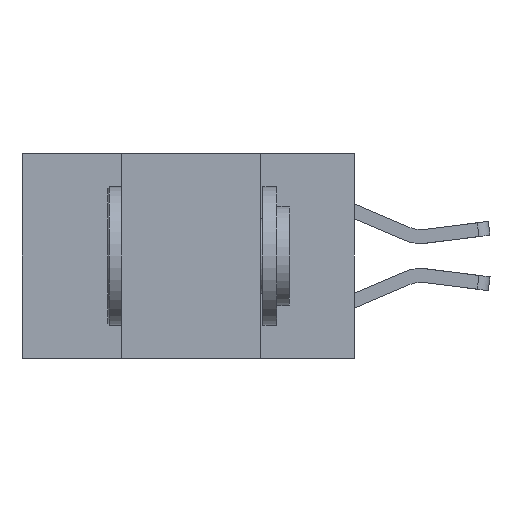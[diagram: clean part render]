
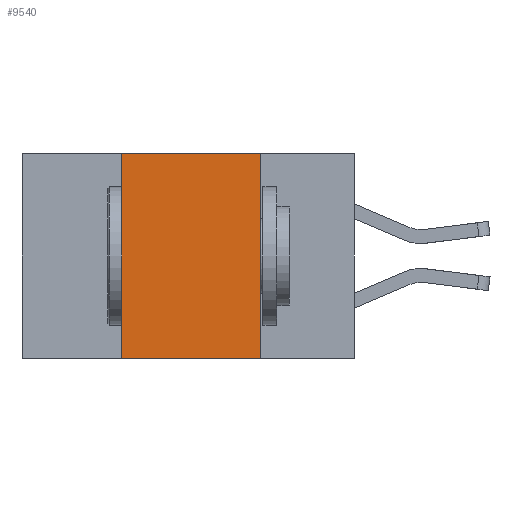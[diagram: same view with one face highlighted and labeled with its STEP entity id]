
A CAD part, left-side view. The second image highlights one B-rep face of the part: STEP entity #9540.
In plain terms, the highlighted planar face has unit normal (-1, 0, 0).
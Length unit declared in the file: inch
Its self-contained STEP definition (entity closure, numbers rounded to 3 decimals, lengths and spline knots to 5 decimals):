
#152 = EDGE_CURVE ( 'NONE', #859, #7637, #5741, .T. ) ;
#662 = EDGE_LOOP ( 'NONE', ( #2563, #6966, #4535, #7061 ) ) ;
#859 = VERTEX_POINT ( 'NONE', #6624 ) ;
#1360 = EDGE_CURVE ( 'NONE', #7637, #4985, #1801, .T. ) ;
#1801 = LINE ( 'NONE', #8387, #7916 ) ;
#1902 = LINE ( 'NONE', #7557, #3897 ) ;
#2563 = ORIENTED_EDGE ( 'NONE', *, *, #4761, .F. ) ;
#2686 = CARTESIAN_POINT ( 'NONE',  ( 0., 0.6, 0. ) ) ;
#2719 = DIRECTION ( 'NONE',  ( 0., 0., -1. ) ) ;
#2731 = AXIS2_PLACEMENT_3D ( 'NONE', #2686, #7675, #2719 ) ;
#3028 = EDGE_CURVE ( 'NONE', #859, #6926, #1902, .T. ) ;
#3897 = VECTOR ( 'NONE', #7527, 39.37008 ) ;
#4080 = VECTOR ( 'NONE', #9337, 39.37008 ) ;
#4535 = ORIENTED_EDGE ( 'NONE', *, *, #152, .F. ) ;
#4761 = EDGE_CURVE ( 'NONE', #4985, #6926, #6246, .T. ) ;
#4819 = DIRECTION ( 'NONE',  ( 0., 0., 1. ) ) ;
#4985 = VERTEX_POINT ( 'NONE', #6222 ) ;
#5354 = DIRECTION ( 'NONE',  ( 0., -1., 0. ) ) ;
#5741 = LINE ( 'NONE', #10121, #7667 ) ;
#6222 = CARTESIAN_POINT ( 'NONE',  ( 0., 0.17, 0. ) ) ;
#6246 = LINE ( 'NONE', #9583, #4080 ) ;
#6279 = CARTESIAN_POINT ( 'NONE',  ( 0., 0.42, 0. ) ) ;
#6624 = CARTESIAN_POINT ( 'NONE',  ( 0., 0.42, -0.37 ) ) ;
#6926 = VERTEX_POINT ( 'NONE', #10239 ) ;
#6966 = ORIENTED_EDGE ( 'NONE', *, *, #1360, .F. ) ;
#7061 = ORIENTED_EDGE ( 'NONE', *, *, #3028, .T. ) ;
#7527 = DIRECTION ( 'NONE',  ( 0., -1., 0. ) ) ;
#7557 = CARTESIAN_POINT ( 'NONE',  ( 0., 0.6, -0.37 ) ) ;
#7637 = VERTEX_POINT ( 'NONE', #6279 ) ;
#7667 = VECTOR ( 'NONE', #4819, 39.37008 ) ;
#7675 = DIRECTION ( 'NONE',  ( 1., 0., 0. ) ) ;
#7916 = VECTOR ( 'NONE', #5354, 39.37008 ) ;
#8387 = CARTESIAN_POINT ( 'NONE',  ( 0., 0.6, 0. ) ) ;
#8426 = PLANE ( 'NONE',  #2731 ) ;
#9337 = DIRECTION ( 'NONE',  ( 0., 0., -1. ) ) ;
#9540 = ADVANCED_FACE ( 'NONE', ( #10163 ), #8426, .F. ) ;
#9583 = CARTESIAN_POINT ( 'NONE',  ( 0., 0.17, -0.37 ) ) ;
#10121 = CARTESIAN_POINT ( 'NONE',  ( 0., 0.42, -0.37 ) ) ;
#10163 = FACE_OUTER_BOUND ( 'NONE', #662, .T. ) ;
#10239 = CARTESIAN_POINT ( 'NONE',  ( 0., 0.17, -0.37 ) ) ;
